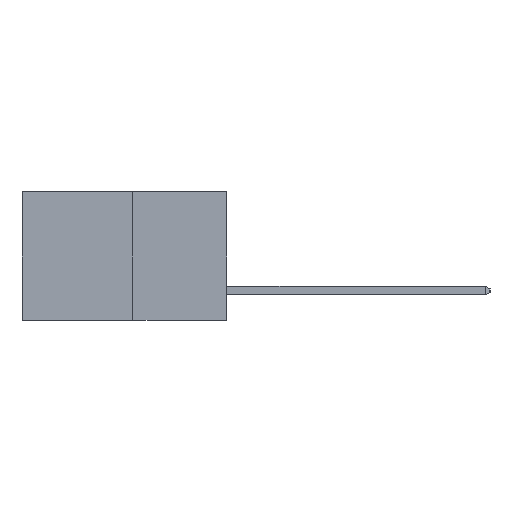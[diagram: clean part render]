
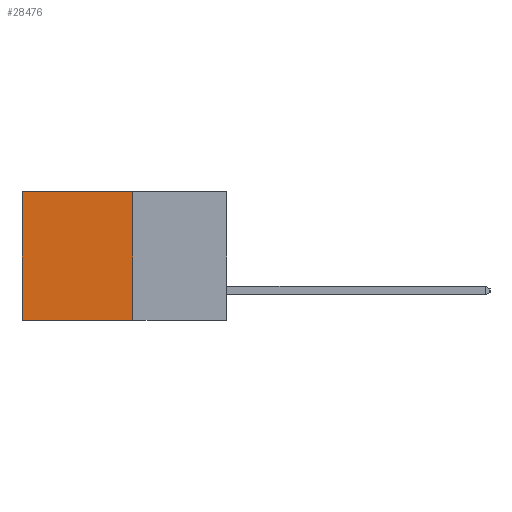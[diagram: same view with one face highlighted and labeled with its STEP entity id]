
A CAD part, left-side view. The second image highlights one B-rep face of the part: STEP entity #28476.
In plain terms, the highlighted planar face has unit normal (-1, 0, 0).
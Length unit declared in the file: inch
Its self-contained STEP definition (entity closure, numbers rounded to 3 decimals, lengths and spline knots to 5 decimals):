
#208 = ORIENTED_EDGE ( 'NONE', *, *, #7372, .T. ) ;
#3093 = VECTOR ( 'NONE', #30838, 39.37008 ) ;
#3467 = EDGE_CURVE ( 'NONE', #9556, #11038, #29922, .T. ) ;
#6334 = CARTESIAN_POINT ( 'NONE',  ( 0.277, 0.27, -0.37 ) ) ;
#7118 = PLANE ( 'NONE',  #27781 ) ;
#7372 = EDGE_CURVE ( 'NONE', #11038, #18522, #28754, .T. ) ;
#8221 = VECTOR ( 'NONE', #16504, 39.37008 ) ;
#9556 = VERTEX_POINT ( 'NONE', #18921 ) ;
#10947 = CARTESIAN_POINT ( 'NONE',  ( 0.277, 0.27, -0.37 ) ) ;
#11038 = VERTEX_POINT ( 'NONE', #27183 ) ;
#12284 = DIRECTION ( 'NONE',  ( 1., 0., 0. ) ) ;
#12873 = CARTESIAN_POINT ( 'NONE',  ( 0.277, 0.27, -0.37 ) ) ;
#15243 = LINE ( 'NONE', #12873, #3093 ) ;
#15778 = ORIENTED_EDGE ( 'NONE', *, *, #3467, .T. ) ;
#16035 = ORIENTED_EDGE ( 'NONE', *, *, #18588, .F. ) ;
#16466 = CARTESIAN_POINT ( 'NONE',  ( 0.277, 0.59, -0.37 ) ) ;
#16504 = DIRECTION ( 'NONE',  ( 0., 0., -1. ) ) ;
#18522 = VERTEX_POINT ( 'NONE', #31708 ) ;
#18588 = EDGE_CURVE ( 'NONE', #22208, #18522, #27099, .T. ) ;
#18921 = CARTESIAN_POINT ( 'NONE',  ( 0.277, 0.27, 0. ) ) ;
#21645 = EDGE_LOOP ( 'NONE', ( #208, #16035, #32017, #15778 ) ) ;
#22208 = VERTEX_POINT ( 'NONE', #10947 ) ;
#22744 = FACE_OUTER_BOUND ( 'NONE', #21645, .T. ) ;
#23107 = VECTOR ( 'NONE', #27788, 39.37008 ) ;
#25149 = CARTESIAN_POINT ( 'NONE',  ( 0.277, 0.27, -0.37 ) ) ;
#26983 = DIRECTION ( 'NONE',  ( 0., 1., 0. ) ) ;
#27099 = LINE ( 'NONE', #6334, #32931 ) ;
#27183 = CARTESIAN_POINT ( 'NONE',  ( 0.277, 0.59, 0. ) ) ;
#27781 = AXIS2_PLACEMENT_3D ( 'NONE', #25149, #12284, #30291 ) ;
#27788 = DIRECTION ( 'NONE',  ( 0., 1., 0. ) ) ;
#27960 = CARTESIAN_POINT ( 'NONE',  ( 0.277, 0.27, 0. ) ) ;
#28476 = ADVANCED_FACE ( 'NONE', ( #22744 ), #7118, .F. ) ;
#28754 = LINE ( 'NONE', #16466, #8221 ) ;
#29922 = LINE ( 'NONE', #27960, #23107 ) ;
#30291 = DIRECTION ( 'NONE',  ( 0., 0., -1. ) ) ;
#30625 = EDGE_CURVE ( 'NONE', #9556, #22208, #15243, .T. ) ;
#30838 = DIRECTION ( 'NONE',  ( 0., 0., -1. ) ) ;
#31708 = CARTESIAN_POINT ( 'NONE',  ( 0.277, 0.59, -0.37 ) ) ;
#32017 = ORIENTED_EDGE ( 'NONE', *, *, #30625, .F. ) ;
#32931 = VECTOR ( 'NONE', #26983, 39.37008 ) ;
